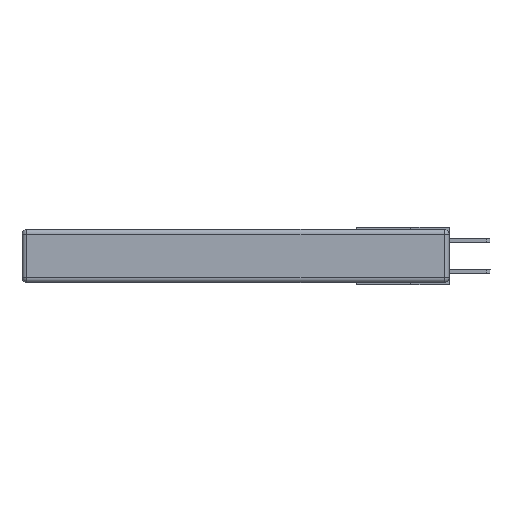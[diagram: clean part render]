
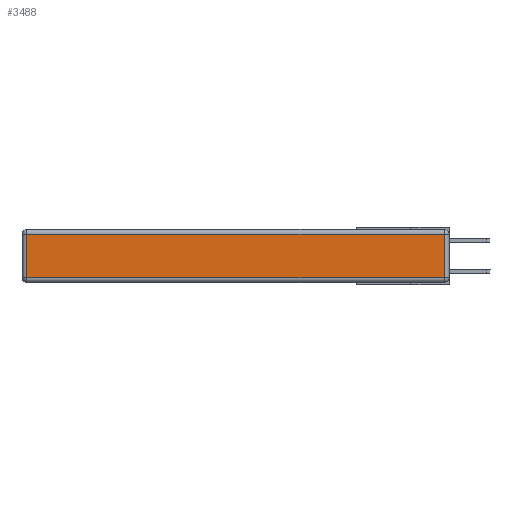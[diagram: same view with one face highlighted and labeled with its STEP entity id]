
A CAD part, left-side view. The second image highlights one B-rep face of the part: STEP entity #3488.
In plain terms, the highlighted planar face has unit normal (-1, 0, 0).
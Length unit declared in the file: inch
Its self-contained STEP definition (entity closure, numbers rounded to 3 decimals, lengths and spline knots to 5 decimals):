
#520 = AXIS2_PLACEMENT_3D ( 'NONE', #10540, #4772, #4736 ) ;
#788 = VERTEX_POINT ( 'NONE', #4131 ) ;
#1218 = VERTEX_POINT ( 'NONE', #5656 ) ;
#1323 = EDGE_CURVE ( 'NONE', #4675, #10614, #10912, .T. ) ;
#1405 = EDGE_CURVE ( 'NONE', #1218, #4675, #6038, .T. ) ;
#1826 = CARTESIAN_POINT ( 'NONE',  ( 0., 2.72, -0.343 ) ) ;
#2740 = DIRECTION ( 'NONE',  ( 0., 0., -1. ) ) ;
#2907 = PLANE ( 'NONE',  #520 ) ;
#2946 = DIRECTION ( 'NONE',  ( 0., 1., 0. ) ) ;
#3488 = ADVANCED_FACE ( 'NONE', ( #4025 ), #2907, .T. ) ;
#3612 = VECTOR ( 'NONE', #12174, 39.37008 ) ;
#3650 = CARTESIAN_POINT ( 'NONE',  ( 0., 0.03, -0.03 ) ) ;
#4025 = FACE_OUTER_BOUND ( 'NONE', #10407, .T. ) ;
#4051 = LINE ( 'NONE', #1826, #8453 ) ;
#4131 = CARTESIAN_POINT ( 'NONE',  ( 0., 2.72, -0.313 ) ) ;
#4675 = VERTEX_POINT ( 'NONE', #3650 ) ;
#4682 = LINE ( 'NONE', #7281, #3612 ) ;
#4736 = DIRECTION ( 'NONE',  ( 0., 0., 1. ) ) ;
#4767 = DIRECTION ( 'NONE',  ( 0., 0., 1. ) ) ;
#4772 = DIRECTION ( 'NONE',  ( -1., 0., 0. ) ) ;
#5656 = CARTESIAN_POINT ( 'NONE',  ( 0., 0.03, -0.313 ) ) ;
#5755 = ORIENTED_EDGE ( 'NONE', *, *, #8164, .T. ) ;
#6038 = LINE ( 'NONE', #10579, #8624 ) ;
#7281 = CARTESIAN_POINT ( 'NONE',  ( 0., 0., -0.313 ) ) ;
#7502 = CARTESIAN_POINT ( 'NONE',  ( 0., 2.72, -0.03 ) ) ;
#7882 = EDGE_CURVE ( 'NONE', #788, #1218, #4682, .T. ) ;
#8148 = ORIENTED_EDGE ( 'NONE', *, *, #1323, .T. ) ;
#8164 = EDGE_CURVE ( 'NONE', #10614, #788, #4051, .T. ) ;
#8453 = VECTOR ( 'NONE', #2740, 39.37008 ) ;
#8624 = VECTOR ( 'NONE', #4767, 39.37008 ) ;
#8667 = CARTESIAN_POINT ( 'NONE',  ( 0., 2.75, -0.03 ) ) ;
#9053 = ORIENTED_EDGE ( 'NONE', *, *, #7882, .T. ) ;
#10275 = ORIENTED_EDGE ( 'NONE', *, *, #1405, .T. ) ;
#10407 = EDGE_LOOP ( 'NONE', ( #9053, #10275, #8148, #5755 ) ) ;
#10540 = CARTESIAN_POINT ( 'NONE',  ( 0., 0., -0.343 ) ) ;
#10579 = CARTESIAN_POINT ( 'NONE',  ( 0., 0.03, -0.343 ) ) ;
#10611 = VECTOR ( 'NONE', #2946, 39.37008 ) ;
#10614 = VERTEX_POINT ( 'NONE', #7502 ) ;
#10912 = LINE ( 'NONE', #8667, #10611 ) ;
#12174 = DIRECTION ( 'NONE',  ( 0., -1., 0. ) ) ;
